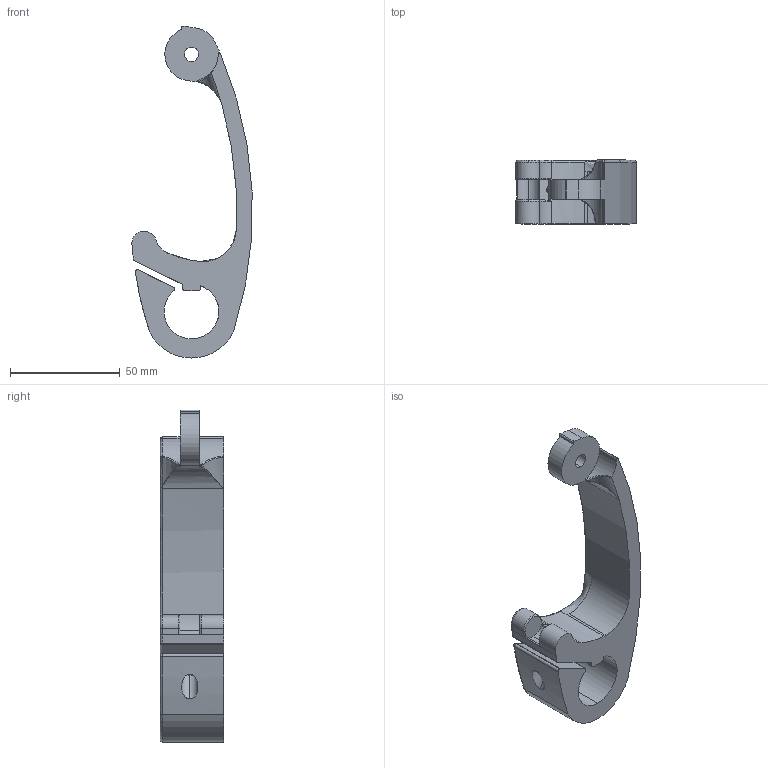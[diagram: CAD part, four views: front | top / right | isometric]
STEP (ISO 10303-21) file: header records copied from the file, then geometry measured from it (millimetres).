
FILE_DESCRIPTION (( 'STEP AP214' ), '1' );
FILE_NAME ('TailhookA.STEP', '2022-08-05T18:42:13', ( '' ), ( '' ), 'SwSTEP 2.0', 'SolidWorks 2021', '' );
FILE_SCHEMA (( 'AUTOMOTIVE_DESIGN' ));
Length unit declared in the file: millimetre
Products named in the file (1): TailhookA
Bounding box: 54.68 x 29 x 151.06 mm (x, y, z)
Volume: 65189.9 mm3; surface area: 20039.3 mm2
Topology: 1 solids, 1 shells, 111 faces, 284 edges, 169 vertices
Faces by surface type: cylinder 55, torus 26, plane 17, bspline 7, sphere 6
Entity records: 5941 total; most frequent: CARTESIAN_POINT 2966, DIRECTION 595, ORIENTED_EDGE 554, EDGE_CURVE 277, AXIS2_PLACEMENT_3D 254, VERTEX_POINT 169, CIRCLE 149, EDGE_LOOP 118
